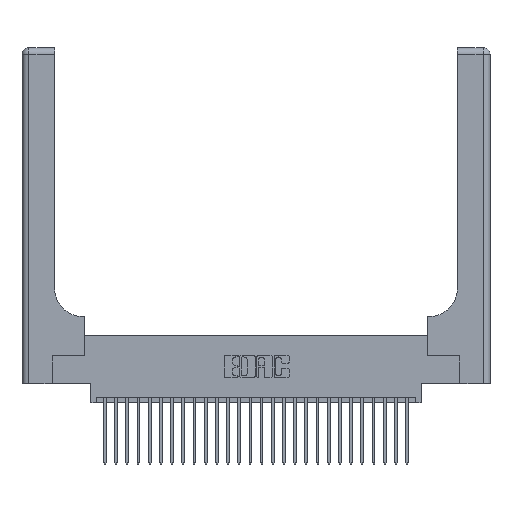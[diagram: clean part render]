
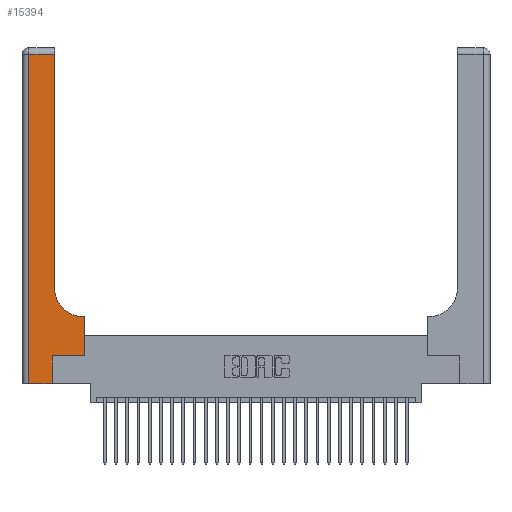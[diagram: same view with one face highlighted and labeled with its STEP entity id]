
A CAD part, top view. The second image highlights one B-rep face of the part: STEP entity #15394.
In plain terms, the highlighted planar face has unit normal (0, 0, 1).
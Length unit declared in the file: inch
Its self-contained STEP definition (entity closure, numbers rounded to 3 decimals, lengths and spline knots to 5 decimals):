
#252 = VECTOR ( 'NONE', #7153, 39.37008 ) ;
#342 = DIRECTION ( 'NONE',  ( 0., 1., 0. ) ) ;
#586 = ORIENTED_EDGE ( 'NONE', *, *, #8156, .T. ) ;
#979 = LINE ( 'NONE', #9306, #252 ) ;
#1021 = CARTESIAN_POINT ( 'NONE',  ( 0.2915, 0.85, 0.37 ) ) ;
#1324 = CARTESIAN_POINT ( 'NONE',  ( 0.06, 2.94, 0.37 ) ) ;
#2859 = LINE ( 'NONE', #22838, #21929 ) ;
#3282 = VECTOR ( 'NONE', #17495, 39.37008 ) ;
#3574 = CARTESIAN_POINT ( 'NONE',  ( 0.2915, 2.94, 0.37 ) ) ;
#3678 = CARTESIAN_POINT ( 'NONE',  ( 0.269, 0., 0.37 ) ) ;
#3959 = VERTEX_POINT ( 'NONE', #24865 ) ;
#3995 = VECTOR ( 'NONE', #29087, 39.37008 ) ;
#4148 = ORIENTED_EDGE ( 'NONE', *, *, #9615, .T. ) ;
#4327 = ORIENTED_EDGE ( 'NONE', *, *, #11630, .T. ) ;
#4515 = VECTOR ( 'NONE', #8434, 39.37008 ) ;
#4561 = CARTESIAN_POINT ( 'NONE',  ( 0.269, 0., 0.37 ) ) ;
#4722 = VERTEX_POINT ( 'NONE', #19825 ) ;
#4782 = ORIENTED_EDGE ( 'NONE', *, *, #27552, .T. ) ;
#5203 = DIRECTION ( 'NONE',  ( -1., 0., 0. ) ) ;
#5931 = DIRECTION ( 'NONE',  ( 1., 0., 0. ) ) ;
#6806 = ORIENTED_EDGE ( 'NONE', *, *, #7005, .T. ) ;
#7005 = EDGE_CURVE ( 'NONE', #14496, #16769, #14611, .T. ) ;
#7153 = DIRECTION ( 'NONE',  ( 1., 0., 0. ) ) ;
#7365 = DIRECTION ( 'NONE',  ( 0., -1., 0. ) ) ;
#8156 = EDGE_CURVE ( 'NONE', #21900, #21809, #19708, .T. ) ;
#8434 = DIRECTION ( 'NONE',  ( 0., 1., 0. ) ) ;
#9305 = LINE ( 'NONE', #19939, #3282 ) ;
#9306 = CARTESIAN_POINT ( 'NONE',  ( 0.269, 0.25, 0.37 ) ) ;
#9615 = EDGE_CURVE ( 'NONE', #12950, #21900, #28705, .T. ) ;
#11006 = VECTOR ( 'NONE', #5931, 39.37008 ) ;
#11630 = EDGE_CURVE ( 'NONE', #4722, #25678, #18740, .T. ) ;
#12207 = FACE_OUTER_BOUND ( 'NONE', #14881, .T. ) ;
#12243 = CARTESIAN_POINT ( 'NONE',  ( 0.5585, 0.6, 0.37 ) ) ;
#12355 = AXIS2_PLACEMENT_3D ( 'NONE', #20664, #25384, #5203 ) ;
#12750 = VECTOR ( 'NONE', #13798, 39.37008 ) ;
#12950 = VERTEX_POINT ( 'NONE', #21800 ) ;
#13563 = CARTESIAN_POINT ( 'NONE',  ( 0.5585, 0.25, 0.37 ) ) ;
#13798 = DIRECTION ( 'NONE',  ( -1., 0., 0. ) ) ;
#14496 = VERTEX_POINT ( 'NONE', #17978 ) ;
#14611 = LINE ( 'NONE', #13563, #3995 ) ;
#14750 = ORIENTED_EDGE ( 'NONE', *, *, #23281, .T. ) ;
#14881 = EDGE_LOOP ( 'NONE', ( #586, #14750, #23912, #4327, #19996, #4782, #6806, #17136, #4148 ) ) ;
#15394 = ADVANCED_FACE ( 'NONE', ( #12207 ), #23143, .F. ) ;
#16769 = VERTEX_POINT ( 'NONE', #12243 ) ;
#17136 = ORIENTED_EDGE ( 'NONE', *, *, #17927, .T. ) ;
#17156 = CARTESIAN_POINT ( 'NONE',  ( 0., 0., 0.37 ) ) ;
#17495 = DIRECTION ( 'NONE',  ( -1., 0., 0. ) ) ;
#17927 = EDGE_CURVE ( 'NONE', #16769, #12950, #18757, .T. ) ;
#17978 = CARTESIAN_POINT ( 'NONE',  ( 0.5585, 0.25, 0.37 ) ) ;
#18331 = EDGE_CURVE ( 'NONE', #22734, #4722, #2859, .T. ) ;
#18740 = LINE ( 'NONE', #17156, #11006 ) ;
#18757 = LINE ( 'NONE', #25020, #12750 ) ;
#19708 = LINE ( 'NONE', #20670, #28153 ) ;
#19825 = CARTESIAN_POINT ( 'NONE',  ( 0.06, 0., 0.37 ) ) ;
#19939 = CARTESIAN_POINT ( 'NONE',  ( 0., 2.94, 0.37 ) ) ;
#19996 = ORIENTED_EDGE ( 'NONE', *, *, #27341, .T. ) ;
#20664 = CARTESIAN_POINT ( 'NONE',  ( 0., 3., 0.37 ) ) ;
#20670 = CARTESIAN_POINT ( 'NONE',  ( 0.2915, 3., 0.37 ) ) ;
#21800 = CARTESIAN_POINT ( 'NONE',  ( 0.5415, 0.6, 0.37 ) ) ;
#21809 = VERTEX_POINT ( 'NONE', #3574 ) ;
#21900 = VERTEX_POINT ( 'NONE', #1021 ) ;
#21929 = VECTOR ( 'NONE', #7365, 39.37008 ) ;
#22522 = LINE ( 'NONE', #3678, #4515 ) ;
#22734 = VERTEX_POINT ( 'NONE', #1324 ) ;
#22838 = CARTESIAN_POINT ( 'NONE',  ( 0.06, 3., 0.37 ) ) ;
#23143 = PLANE ( 'NONE',  #12355 ) ;
#23281 = EDGE_CURVE ( 'NONE', #21809, #22734, #9305, .T. ) ;
#23912 = ORIENTED_EDGE ( 'NONE', *, *, #18331, .T. ) ;
#24865 = CARTESIAN_POINT ( 'NONE',  ( 0.269, 0.25, 0.37 ) ) ;
#24934 = CARTESIAN_POINT ( 'NONE',  ( 0.5415, 0.85, 0.37 ) ) ;
#25020 = CARTESIAN_POINT ( 'NONE',  ( 0.2915, 0.6, 0.37 ) ) ;
#25384 = DIRECTION ( 'NONE',  ( 0., 0., -1. ) ) ;
#25678 = VERTEX_POINT ( 'NONE', #4561 ) ;
#25784 = AXIS2_PLACEMENT_3D ( 'NONE', #24934, #27271, #26968 ) ;
#26968 = DIRECTION ( 'NONE',  ( 1., 0., 0. ) ) ;
#27271 = DIRECTION ( 'NONE',  ( 0., 0., -1. ) ) ;
#27341 = EDGE_CURVE ( 'NONE', #25678, #3959, #22522, .T. ) ;
#27552 = EDGE_CURVE ( 'NONE', #3959, #14496, #979, .T. ) ;
#28153 = VECTOR ( 'NONE', #342, 39.37008 ) ;
#28705 = CIRCLE ( 'NONE', #25784, 0.25 ) ;
#29087 = DIRECTION ( 'NONE',  ( 0., 1., 0. ) ) ;
